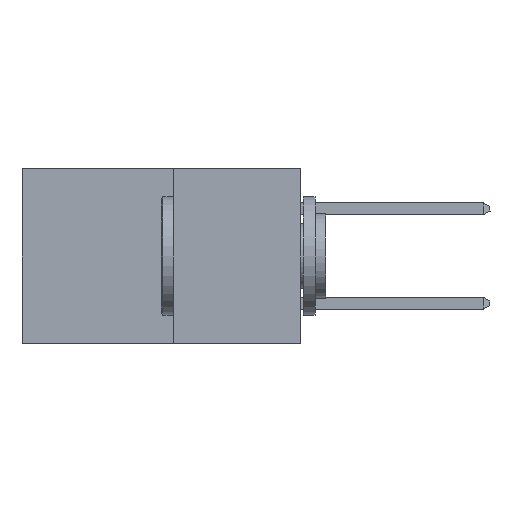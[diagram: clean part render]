
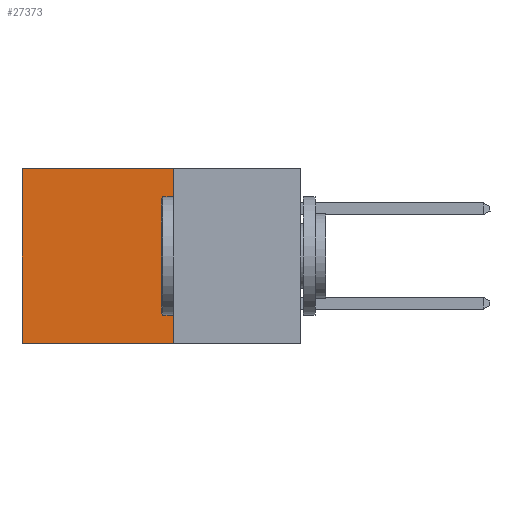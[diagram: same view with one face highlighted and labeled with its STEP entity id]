
A CAD part, left-side view. The second image highlights one B-rep face of the part: STEP entity #27373.
In plain terms, the highlighted planar face has unit normal (-1, 0, 0).
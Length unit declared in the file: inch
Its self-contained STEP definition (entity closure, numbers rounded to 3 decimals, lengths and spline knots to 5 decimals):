
#108 = FACE_OUTER_BOUND ( 'NONE', #26173, .T. ) ;
#320 = VECTOR ( 'NONE', #19405, 39.37008 ) ;
#1985 = ORIENTED_EDGE ( 'NONE', *, *, #6077, .T. ) ;
#3406 = VERTEX_POINT ( 'NONE', #15683 ) ;
#5443 = CARTESIAN_POINT ( 'NONE',  ( 0.277, 0.27, 0. ) ) ;
#6077 = EDGE_CURVE ( 'NONE', #3406, #8244, #25621, .T. ) ;
#6193 = VECTOR ( 'NONE', #13273, 39.37008 ) ;
#8244 = VERTEX_POINT ( 'NONE', #16435 ) ;
#8637 = VERTEX_POINT ( 'NONE', #5443 ) ;
#8865 = PLANE ( 'NONE',  #9112 ) ;
#9112 = AXIS2_PLACEMENT_3D ( 'NONE', #25932, #28373, #13817 ) ;
#9295 = LINE ( 'NONE', #10701, #6193 ) ;
#10701 = CARTESIAN_POINT ( 'NONE',  ( 0.277, 0.27, -0.37 ) ) ;
#11043 = ORIENTED_EDGE ( 'NONE', *, *, #27195, .T. ) ;
#13273 = DIRECTION ( 'NONE',  ( 0., 0., -1. ) ) ;
#13343 = VECTOR ( 'NONE', #27015, 39.37008 ) ;
#13817 = DIRECTION ( 'NONE',  ( 0., 0., -1. ) ) ;
#14644 = CARTESIAN_POINT ( 'NONE',  ( 0.277, 0.59, -0.37 ) ) ;
#15524 = CARTESIAN_POINT ( 'NONE',  ( 0.277, 0.27, 0. ) ) ;
#15683 = CARTESIAN_POINT ( 'NONE',  ( 0.277, 0.59, 0. ) ) ;
#16435 = CARTESIAN_POINT ( 'NONE',  ( 0.277, 0.59, -0.37 ) ) ;
#19405 = DIRECTION ( 'NONE',  ( 0., 0., -1. ) ) ;
#22420 = ORIENTED_EDGE ( 'NONE', *, *, #25563, .F. ) ;
#22472 = EDGE_CURVE ( 'NONE', #8637, #29554, #9295, .T. ) ;
#23755 = CARTESIAN_POINT ( 'NONE',  ( 0.277, 0.27, -0.37 ) ) ;
#24307 = ORIENTED_EDGE ( 'NONE', *, *, #22472, .F. ) ;
#24580 = CARTESIAN_POINT ( 'NONE',  ( 0.277, 0.27, -0.37 ) ) ;
#25039 = VECTOR ( 'NONE', #30112, 39.37008 ) ;
#25563 = EDGE_CURVE ( 'NONE', #29554, #8244, #26286, .T. ) ;
#25621 = LINE ( 'NONE', #14644, #320 ) ;
#25932 = CARTESIAN_POINT ( 'NONE',  ( 0.277, 0.27, -0.37 ) ) ;
#26173 = EDGE_LOOP ( 'NONE', ( #1985, #22420, #24307, #11043 ) ) ;
#26286 = LINE ( 'NONE', #24580, #13343 ) ;
#27015 = DIRECTION ( 'NONE',  ( 0., 1., 0. ) ) ;
#27195 = EDGE_CURVE ( 'NONE', #8637, #3406, #30765, .T. ) ;
#27373 = ADVANCED_FACE ( 'NONE', ( #108 ), #8865, .F. ) ;
#28373 = DIRECTION ( 'NONE',  ( 1., 0., 0. ) ) ;
#29554 = VERTEX_POINT ( 'NONE', #23755 ) ;
#30112 = DIRECTION ( 'NONE',  ( 0., 1., 0. ) ) ;
#30765 = LINE ( 'NONE', #15524, #25039 ) ;
